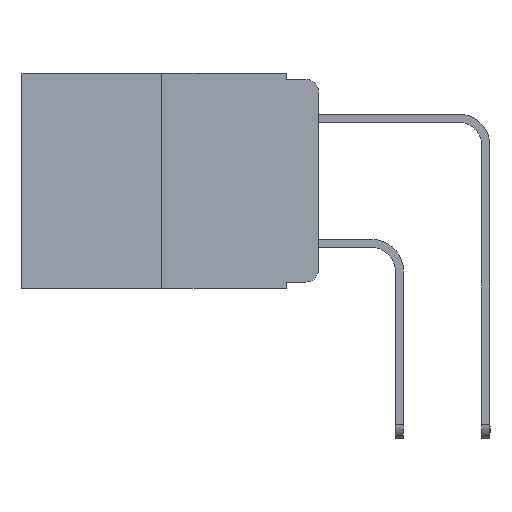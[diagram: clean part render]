
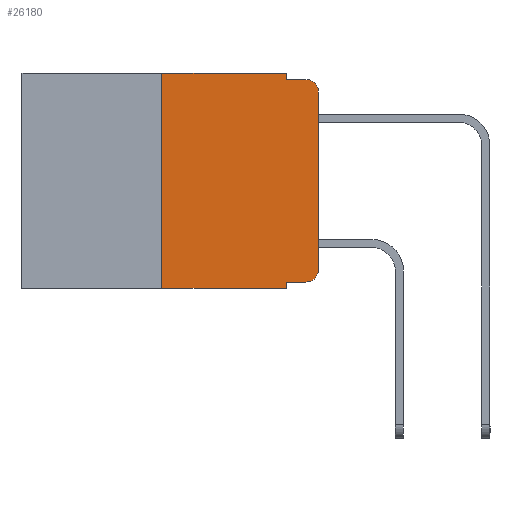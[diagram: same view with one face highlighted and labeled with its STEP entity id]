
A CAD part, left-side view. The second image highlights one B-rep face of the part: STEP entity #26180.
In plain terms, the highlighted planar face has unit normal (-1, 0, 0).
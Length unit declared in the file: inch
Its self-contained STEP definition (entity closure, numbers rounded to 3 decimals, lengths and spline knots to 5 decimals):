
#193 = AXIS2_PLACEMENT_3D ( 'NONE', #9565, #24599, #5348 ) ;
#292 = EDGE_CURVE ( 'NONE', #10817, #20532, #16048, .T. ) ;
#463 = ORIENTED_EDGE ( 'NONE', *, *, #8252, .F. ) ;
#635 = AXIS2_PLACEMENT_3D ( 'NONE', #21300, #6544, #6256 ) ;
#728 = VERTEX_POINT ( 'NONE', #20230 ) ;
#951 = VECTOR ( 'NONE', #11137, 39.37008 ) ;
#1198 = LINE ( 'NONE', #5134, #16504 ) ;
#1199 = LINE ( 'NONE', #5551, #20970 ) ;
#1364 = DIRECTION ( 'NONE',  ( 0., 0., 1. ) ) ;
#1519 = FACE_OUTER_BOUND ( 'NONE', #26137, .T. ) ;
#1911 = VERTEX_POINT ( 'NONE', #15092 ) ;
#2494 = LINE ( 'NONE', #12771, #19016 ) ;
#2712 = ORIENTED_EDGE ( 'NONE', *, *, #292, .T. ) ;
#2897 = EDGE_CURVE ( 'NONE', #728, #15997, #1198, .T. ) ;
#3096 = LINE ( 'NONE', #6908, #951 ) ;
#3158 = DIRECTION ( 'NONE',  ( 0., -1., 0. ) ) ;
#3476 = ORIENTED_EDGE ( 'NONE', *, *, #5331, .F. ) ;
#3772 = VERTEX_POINT ( 'NONE', #8425 ) ;
#3956 = EDGE_CURVE ( 'NONE', #20532, #13301, #12302, .T. ) ;
#5134 = CARTESIAN_POINT ( 'NONE',  ( 0., 0.473, -0.343 ) ) ;
#5331 = EDGE_CURVE ( 'NONE', #728, #3772, #16120, .T. ) ;
#5348 = DIRECTION ( 'NONE',  ( 0., 0., -1. ) ) ;
#5402 = CARTESIAN_POINT ( 'NONE',  ( 0., 0., 0. ) ) ;
#5421 = VECTOR ( 'NONE', #22647, 39.37008 ) ;
#5550 = DIRECTION ( 'NONE',  ( 0., -1., 0. ) ) ;
#5551 = CARTESIAN_POINT ( 'NONE',  ( 0., 0.051, -0.01 ) ) ;
#5562 = ORIENTED_EDGE ( 'NONE', *, *, #13879, .T. ) ;
#5595 = PLANE ( 'NONE',  #11895 ) ;
#6101 = CARTESIAN_POINT ( 'NONE',  ( 0., 0.473, 0. ) ) ;
#6256 = DIRECTION ( 'NONE',  ( 0., 0., -1. ) ) ;
#6544 = DIRECTION ( 'NONE',  ( -1., 0., 0. ) ) ;
#6635 = VERTEX_POINT ( 'NONE', #13620 ) ;
#6908 = CARTESIAN_POINT ( 'NONE',  ( 0., 0.051, 0. ) ) ;
#7129 = EDGE_CURVE ( 'NONE', #1911, #6635, #1199, .T. ) ;
#8252 = EDGE_CURVE ( 'NONE', #3772, #12463, #27737, .T. ) ;
#8273 = DIRECTION ( 'NONE',  ( 1., 0., 0. ) ) ;
#8425 = CARTESIAN_POINT ( 'NONE',  ( 0., 0.25, 0. ) ) ;
#8444 = VERTEX_POINT ( 'NONE', #11302 ) ;
#8449 = VECTOR ( 'NONE', #10618, 39.37008 ) ;
#9222 = CARTESIAN_POINT ( 'NONE',  ( 0., 0.051, 0. ) ) ;
#9565 = CARTESIAN_POINT ( 'NONE',  ( 0., 0.02, -0.03 ) ) ;
#10618 = DIRECTION ( 'NONE',  ( 0., -1., 0. ) ) ;
#10817 = VERTEX_POINT ( 'NONE', #17833 ) ;
#11137 = DIRECTION ( 'NONE',  ( 0., 0., -1. ) ) ;
#11229 = CARTESIAN_POINT ( 'NONE',  ( 0., 0., -0.313 ) ) ;
#11302 = CARTESIAN_POINT ( 'NONE',  ( 0., 0., -0.03 ) ) ;
#11895 = AXIS2_PLACEMENT_3D ( 'NONE', #20491, #8273, #16410 ) ;
#11924 = CARTESIAN_POINT ( 'NONE',  ( 0., 0.25, 0. ) ) ;
#12029 = LINE ( 'NONE', #5402, #15292 ) ;
#12302 = CIRCLE ( 'NONE', #635, 0.02 ) ;
#12463 = VERTEX_POINT ( 'NONE', #9222 ) ;
#12756 = CIRCLE ( 'NONE', #193, 0.02 ) ;
#12771 = CARTESIAN_POINT ( 'NONE',  ( 0., 0.051, 0. ) ) ;
#13301 = VERTEX_POINT ( 'NONE', #11229 ) ;
#13620 = CARTESIAN_POINT ( 'NONE',  ( 0., 0.02, -0.01 ) ) ;
#13879 = EDGE_CURVE ( 'NONE', #13301, #8444, #12029, .T. ) ;
#14088 = CARTESIAN_POINT ( 'NONE',  ( 0., 0.051, -0.333 ) ) ;
#14272 = DIRECTION ( 'NONE',  ( 0., 0., 1. ) ) ;
#15092 = CARTESIAN_POINT ( 'NONE',  ( 0., 0.051, -0.01 ) ) ;
#15292 = VECTOR ( 'NONE', #14272, 39.37008 ) ;
#15885 = ORIENTED_EDGE ( 'NONE', *, *, #7129, .F. ) ;
#15997 = VERTEX_POINT ( 'NONE', #26560 ) ;
#16048 = LINE ( 'NONE', #14088, #5421 ) ;
#16120 = LINE ( 'NONE', #11924, #27606 ) ;
#16290 = ORIENTED_EDGE ( 'NONE', *, *, #17123, .F. ) ;
#16410 = DIRECTION ( 'NONE',  ( 0., 0., -1. ) ) ;
#16504 = VECTOR ( 'NONE', #5550, 39.37008 ) ;
#16651 = ORIENTED_EDGE ( 'NONE', *, *, #25670, .T. ) ;
#17123 = EDGE_CURVE ( 'NONE', #12463, #1911, #3096, .T. ) ;
#17833 = CARTESIAN_POINT ( 'NONE',  ( 0., 0.051, -0.333 ) ) ;
#19016 = VECTOR ( 'NONE', #19225, 39.37008 ) ;
#19225 = DIRECTION ( 'NONE',  ( 0., 0., -1. ) ) ;
#20230 = CARTESIAN_POINT ( 'NONE',  ( 0., 0.25, -0.343 ) ) ;
#20491 = CARTESIAN_POINT ( 'NONE',  ( 0., 0.473, 0. ) ) ;
#20532 = VERTEX_POINT ( 'NONE', #24664 ) ;
#20970 = VECTOR ( 'NONE', #3158, 39.37008 ) ;
#21300 = CARTESIAN_POINT ( 'NONE',  ( 0., 0.02, -0.313 ) ) ;
#22647 = DIRECTION ( 'NONE',  ( 0., -1., 0. ) ) ;
#22673 = ORIENTED_EDGE ( 'NONE', *, *, #3956, .T. ) ;
#23366 = ORIENTED_EDGE ( 'NONE', *, *, #27622, .F. ) ;
#24599 = DIRECTION ( 'NONE',  ( -1., 0., 0. ) ) ;
#24664 = CARTESIAN_POINT ( 'NONE',  ( 0., 0.02, -0.333 ) ) ;
#25670 = EDGE_CURVE ( 'NONE', #8444, #6635, #12756, .T. ) ;
#25841 = ORIENTED_EDGE ( 'NONE', *, *, #2897, .T. ) ;
#26137 = EDGE_LOOP ( 'NONE', ( #5562, #16651, #15885, #16290, #463, #3476, #25841, #23366, #2712, #22673 ) ) ;
#26180 = ADVANCED_FACE ( 'NONE', ( #1519 ), #5595, .F. ) ;
#26560 = CARTESIAN_POINT ( 'NONE',  ( 0., 0.051, -0.343 ) ) ;
#27606 = VECTOR ( 'NONE', #1364, 39.37008 ) ;
#27622 = EDGE_CURVE ( 'NONE', #10817, #15997, #2494, .T. ) ;
#27737 = LINE ( 'NONE', #6101, #8449 ) ;
